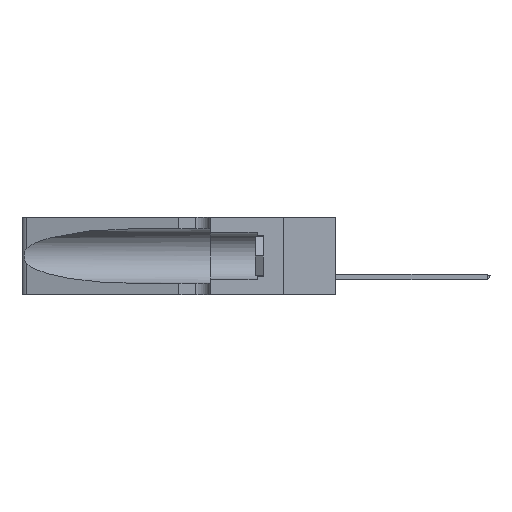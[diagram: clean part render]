
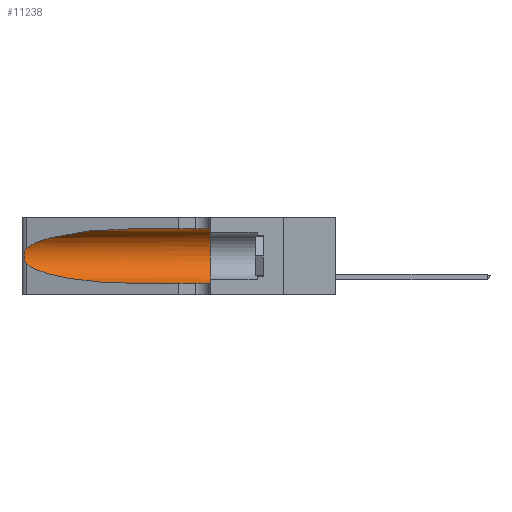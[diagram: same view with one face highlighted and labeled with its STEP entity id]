
A CAD part, left-side view. The second image highlights one B-rep face of the part: STEP entity #11238.
In plain terms, the highlighted cylindrical face has radius 3.308 mm (diameter 6.617 mm), a partial arc.
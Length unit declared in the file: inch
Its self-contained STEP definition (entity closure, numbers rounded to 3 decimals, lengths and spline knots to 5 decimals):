
#795 = CARTESIAN_POINT ( 'NONE',  ( 0.26075, 1.23896, 0.178 ) ) ;
#1446 = CARTESIAN_POINT ( 'NONE',  ( 0.18966, 0.96281, 0.05475 ) ) ;
#2506 = ORIENTED_EDGE ( 'NONE', *, *, #13347, .F. ) ;
#2951 = DIRECTION ( 'NONE',  ( 0., 1., 0. ) ) ;
#3686 = DIRECTION ( 'NONE',  ( 0., 0., -1. ) ) ;
#5459 = CARTESIAN_POINT ( 'NONE',  ( 0.26018, 1.23835, 0.19895 ) ) ;
#5836 = VECTOR ( 'NONE', #46345, 39.37008 ) ;
#6228 = EDGE_LOOP ( 'NONE', ( #11100, #18020, #42621, #41151, #2506, #29242 ) ) ;
#6828 = CARTESIAN_POINT ( 'NONE',  ( 0.1305, 0.72297, 0.31525 ) ) ;
#8101 = LINE ( 'NONE', #42271, #44821 ) ;
#10857 = DIRECTION ( 'NONE',  ( 0., -1., 0. ) ) ;
#11100 = ORIENTED_EDGE ( 'NONE', *, *, #22356, .T. ) ;
#11238 = ADVANCED_FACE ( 'NONE', ( #13006 ), #29881, .F. ) ;
#11513 = DIRECTION ( 'NONE',  ( 0., -1., 0. ) ) ;
#12447 = CARTESIAN_POINT ( 'NONE',  ( 0.26017, 1.23833, 0.17102 ) ) ;
#13006 = FACE_OUTER_BOUND ( 'NONE', #6228, .T. ) ;
#13347 = EDGE_CURVE ( 'NONE', #19881, #36745, #20099, .T. ) ;
#15265 = CARTESIAN_POINT ( 'NONE',  ( 0.25787, 1.23484, 0.2124 ) ) ;
#15400 =( BOUNDED_CURVE ( )  B_SPLINE_CURVE ( 3, ( #6828, #21507, #39661, #18027 ),
 .UNSPECIFIED., .F., .F. ) 
 B_SPLINE_CURVE_WITH_KNOTS ( ( 4, 4 ),
 ( 1.5708, 2.84003 ),
 .UNSPECIFIED. ) 
 CURVE ( )  GEOMETRIC_REPRESENTATION_ITEM ( )  RATIONAL_B_SPLINE_CURVE ( ( 1., 0.87, 0.87, 1. ) ) 
 REPRESENTATION_ITEM ( '' )  );
#16067 = CARTESIAN_POINT ( 'NONE',  ( 0.25856, 1.23593, 0.16098 ) ) ;
#16223 = CARTESIAN_POINT ( 'NONE',  ( 0.25555, 1.22994, 0.2215 ) ) ;
#18020 = ORIENTED_EDGE ( 'NONE', *, *, #39461, .T. ) ;
#18027 = CARTESIAN_POINT ( 'NONE',  ( 0.25487, 1.22718, 0.22369 ) ) ;
#19465 = CARTESIAN_POINT ( 'NONE',  ( 0.1305, 0.72297, 0.31525 ) ) ;
#19533 = CARTESIAN_POINT ( 'NONE',  ( 0.25487, 1.22718, 0.14631 ) ) ;
#19546 = CARTESIAN_POINT ( 'NONE',  ( 0.25487, 1.22718, 0.14631 ) ) ;
#19698 = CARTESIAN_POINT ( 'NONE',  ( 0.25639, 1.23186, 0.15144 ) ) ;
#19881 = VERTEX_POINT ( 'NONE', #45720 ) ;
#20099 = CIRCLE ( 'NONE', #33058, 0.13025 ) ;
#21507 = CARTESIAN_POINT ( 'NONE',  ( 0.18966, 0.96281, 0.31525 ) ) ;
#22220 = EDGE_CURVE ( 'NONE', #23626, #36745, #8101, .T. ) ;
#22356 = EDGE_CURVE ( 'NONE', #26288, #42752, #15400, .T. ) ;
#22478 = CARTESIAN_POINT ( 'NONE',  ( 0.26075, 1.23896, 0.19203 ) ) ;
#23302 = CARTESIAN_POINT ( 'NONE',  ( 0.25487, 1.22718, 0.14631 ) ) ;
#23626 = VERTEX_POINT ( 'NONE', #35197 ) ;
#24048 = VERTEX_POINT ( 'NONE', #19546 ) ;
#26024 = AXIS2_PLACEMENT_3D ( 'NONE', #42625, #10857, #3686 ) ;
#26067 = CARTESIAN_POINT ( 'NONE',  ( 0.1305, 0.35, 0.05475 ) ) ;
#26288 = VERTEX_POINT ( 'NONE', #19465 ) ;
#26761 = CARTESIAN_POINT ( 'NONE',  ( 0.2373, 1.15595, 0.08982 ) ) ;
#27081 = CARTESIAN_POINT ( 'NONE',  ( 0.25639, 1.23184, 0.21858 ) ) ;
#29242 = ORIENTED_EDGE ( 'NONE', *, *, #32348, .F. ) ;
#29881 = CYLINDRICAL_SURFACE ( 'NONE', #26024, 0.13025 ) ;
#31283 = LINE ( 'NONE', #42892, #5836 ) ;
#32348 = EDGE_CURVE ( 'NONE', #26288, #19881, #31283, .T. ) ;
#33058 = AXIS2_PLACEMENT_3D ( 'NONE', #35229, #2951, #42483 ) ;
#35197 = CARTESIAN_POINT ( 'NONE',  ( 0.1305, 0.72297, 0.05475 ) ) ;
#35229 = CARTESIAN_POINT ( 'NONE',  ( 0.1305, 0.35, 0.185 ) ) ;
#36745 = VERTEX_POINT ( 'NONE', #26067 ) ;
#37426 = EDGE_CURVE ( 'NONE', #24048, #23626, #46133, .T. ) ;
#39461 = EDGE_CURVE ( 'NONE', #42752, #24048, #43258, .T. ) ;
#39661 = CARTESIAN_POINT ( 'NONE',  ( 0.2373, 1.15595, 0.28018 ) ) ;
#40510 = CARTESIAN_POINT ( 'NONE',  ( 0.25854, 1.2359, 0.20912 ) ) ;
#40529 = CARTESIAN_POINT ( 'NONE',  ( 0.25487, 1.22718, 0.22369 ) ) ;
#41151 = ORIENTED_EDGE ( 'NONE', *, *, #22220, .T. ) ;
#41348 = CARTESIAN_POINT ( 'NONE',  ( 0.25789, 1.23486, 0.15765 ) ) ;
#42271 = CARTESIAN_POINT ( 'NONE',  ( 0.1305, 1.61858, 0.05475 ) ) ;
#42483 = DIRECTION ( 'NONE',  ( 0., 0., 1. ) ) ;
#42621 = ORIENTED_EDGE ( 'NONE', *, *, #37426, .T. ) ;
#42625 = CARTESIAN_POINT ( 'NONE',  ( 0.1305, 1.61858, 0.185 ) ) ;
#42752 = VERTEX_POINT ( 'NONE', #40529 ) ;
#42892 = CARTESIAN_POINT ( 'NONE',  ( 0.1305, 1.61858, 0.31525 ) ) ;
#43258 = B_SPLINE_CURVE_WITH_KNOTS ( 'NONE', 3,
 ( #45279, #16223, #27081, #15265, #40510, #5459, #22478, #795, #12447, #16067, #41348, #19698, #44939, #23302 ),
 .UNSPECIFIED., .F., .F.,
 ( 4, 2, 2, 2, 2, 2, 4 ),
 ( 0., 0.00027, 0.00053, 0.00107, 0.0016, 0.00187, 0.00214 ),
 .UNSPECIFIED. ) ;
#44629 = CARTESIAN_POINT ( 'NONE',  ( 0.1305, 0.72297, 0.05475 ) ) ;
#44821 = VECTOR ( 'NONE', #11513, 39.37008 ) ;
#44939 = CARTESIAN_POINT ( 'NONE',  ( 0.25555, 1.22993, 0.14849 ) ) ;
#45279 = CARTESIAN_POINT ( 'NONE',  ( 0.25487, 1.22718, 0.22369 ) ) ;
#45720 = CARTESIAN_POINT ( 'NONE',  ( 0.1305, 0.35, 0.31525 ) ) ;
#46133 =( BOUNDED_CURVE ( )  B_SPLINE_CURVE ( 3, ( #19533, #26761, #1446, #44629 ),
 .UNSPECIFIED., .F., .F. ) 
 B_SPLINE_CURVE_WITH_KNOTS ( ( 4, 4 ),
 ( 3.44316, 4.71239 ),
 .UNSPECIFIED. ) 
 CURVE ( )  GEOMETRIC_REPRESENTATION_ITEM ( )  RATIONAL_B_SPLINE_CURVE ( ( 1., 0.87, 0.87, 1. ) ) 
 REPRESENTATION_ITEM ( '' )  );
#46345 = DIRECTION ( 'NONE',  ( 0., -1., 0. ) ) ;
